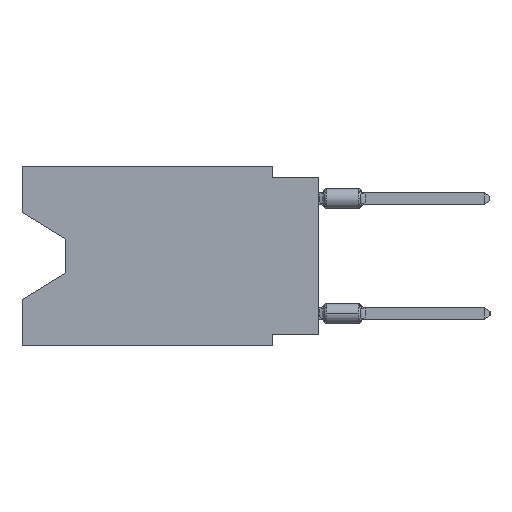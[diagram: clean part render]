
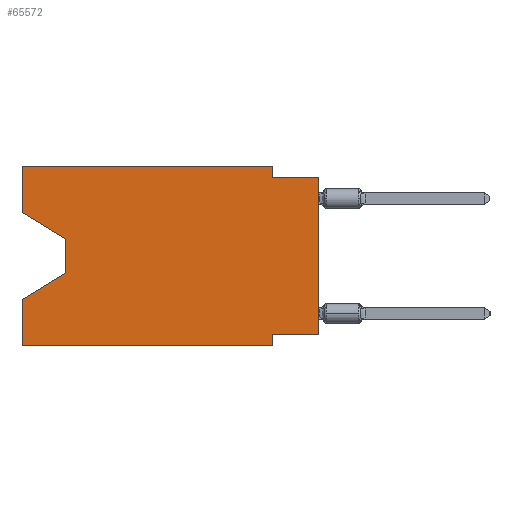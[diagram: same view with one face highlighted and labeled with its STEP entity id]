
A CAD part, left-side view. The second image highlights one B-rep face of the part: STEP entity #65572.
In plain terms, the highlighted planar face has unit normal (-1, 0, 0).
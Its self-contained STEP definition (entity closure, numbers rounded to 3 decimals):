
#178 = VERTEX_POINT ( 'NONE', #41711 ) ;
#434 = EDGE_LOOP ( 'NONE', ( #45684, #6684, #26551, #58628, #59615, #11259, #57603, #14913, #14686, #62036, #37159, #50670 ) ) ;
#535 = VECTOR ( 'NONE', #15756, 1000. ) ;
#4639 = CARTESIAN_POINT ( 'NONE',  ( 0., 2.54, -9.906 ) ) ;
#4961 = VERTEX_POINT ( 'NONE', #57765 ) ;
#5822 = LINE ( 'NONE', #10524, #52215 ) ;
#6130 = VECTOR ( 'NONE', #61492, 1000. ) ;
#6453 = EDGE_CURVE ( 'NONE', #56384, #14442, #25239, .T. ) ;
#6616 = DIRECTION ( 'NONE',  ( 0., 0., 1. ) ) ;
#6684 = ORIENTED_EDGE ( 'NONE', *, *, #17452, .T. ) ;
#6931 = VECTOR ( 'NONE', #47889, 1000. ) ;
#8905 = LINE ( 'NONE', #34385, #12551 ) ;
#10524 = CARTESIAN_POINT ( 'NONE',  ( 0., 16.383, 0. ) ) ;
#11259 = ORIENTED_EDGE ( 'NONE', *, *, #6453, .F. ) ;
#12551 = VECTOR ( 'NONE', #44759, 1000. ) ;
#14379 = VECTOR ( 'NONE', #50388, 1000. ) ;
#14442 = VERTEX_POINT ( 'NONE', #4639 ) ;
#14477 = DIRECTION ( 'NONE',  ( 1., 0., 0. ) ) ;
#14686 = ORIENTED_EDGE ( 'NONE', *, *, #37197, .F. ) ;
#14913 = ORIENTED_EDGE ( 'NONE', *, *, #18314, .T. ) ;
#15156 = EDGE_CURVE ( 'NONE', #62405, #14442, #58585, .T. ) ;
#15756 = DIRECTION ( 'NONE',  ( 0., -0.855, -0.519 ) ) ;
#15877 = DIRECTION ( 'NONE',  ( 0., 0., 1. ) ) ;
#17452 = EDGE_CURVE ( 'NONE', #178, #46009, #27142, .T. ) ;
#17463 = VECTOR ( 'NONE', #6616, 1000. ) ;
#18109 = EDGE_CURVE ( 'NONE', #46009, #28885, #8905, .T. ) ;
#18314 = EDGE_CURVE ( 'NONE', #55580, #65792, #21936, .T. ) ;
#18343 = CARTESIAN_POINT ( 'NONE',  ( 0., 16.383, 0. ) ) ;
#20516 = DIRECTION ( 'NONE',  ( 0., 0., -1. ) ) ;
#21173 = VERTEX_POINT ( 'NONE', #26795 ) ;
#21936 = LINE ( 'NONE', #31014, #6130 ) ;
#22199 = EDGE_CURVE ( 'NONE', #33017, #21173, #59410, .T. ) ;
#23443 = EDGE_CURVE ( 'NONE', #57214, #178, #41226, .T. ) ;
#24512 = VECTOR ( 'NONE', #20516, 1000. ) ;
#25239 = LINE ( 'NONE', #62047, #24512 ) ;
#25458 = CARTESIAN_POINT ( 'NONE',  ( 0., 2.54, 0. ) ) ;
#25638 = CARTESIAN_POINT ( 'NONE',  ( 0., 16.383, -9.906 ) ) ;
#26440 = CARTESIAN_POINT ( 'NONE',  ( 0., 16.383, -7.36 ) ) ;
#26551 = ORIENTED_EDGE ( 'NONE', *, *, #18109, .T. ) ;
#26795 = CARTESIAN_POINT ( 'NONE',  ( 0., 2.54, 0. ) ) ;
#27142 = LINE ( 'NONE', #31824, #30812 ) ;
#28885 = VERTEX_POINT ( 'NONE', #26440 ) ;
#29266 = CARTESIAN_POINT ( 'NONE',  ( 0., 16.383, 0. ) ) ;
#30488 = LINE ( 'NONE', #25458, #59385 ) ;
#30620 = DIRECTION ( 'NONE',  ( 0., -1., 0. ) ) ;
#30709 = CARTESIAN_POINT ( 'NONE',  ( 0., 2.54, -9.271 ) ) ;
#30812 = VECTOR ( 'NONE', #47907, 1000. ) ;
#31014 = CARTESIAN_POINT ( 'NONE',  ( 0., 0., 0. ) ) ;
#31824 = CARTESIAN_POINT ( 'NONE',  ( 0., 13.97, -4.013 ) ) ;
#33017 = VERTEX_POINT ( 'NONE', #18343 ) ;
#33186 = VECTOR ( 'NONE', #30620, 1000. ) ;
#34385 = CARTESIAN_POINT ( 'NONE',  ( 0., 13.97, -5.893 ) ) ;
#36876 = CARTESIAN_POINT ( 'NONE',  ( 0., 0., -0.635 ) ) ;
#37159 = ORIENTED_EDGE ( 'NONE', *, *, #22199, .F. ) ;
#37197 = EDGE_CURVE ( 'NONE', #4961, #65792, #61743, .T. ) ;
#37778 = CARTESIAN_POINT ( 'NONE',  ( 0., 16.383, 0. ) ) ;
#40030 = CARTESIAN_POINT ( 'NONE',  ( 0., 13.97, -5.893 ) ) ;
#41226 = LINE ( 'NONE', #42213, #535 ) ;
#41711 = CARTESIAN_POINT ( 'NONE',  ( 0., 13.97, -4.013 ) ) ;
#42213 = CARTESIAN_POINT ( 'NONE',  ( 0., 16.383, -2.546 ) ) ;
#42941 = EDGE_CURVE ( 'NONE', #62405, #28885, #47854, .T. ) ;
#43161 = CARTESIAN_POINT ( 'NONE',  ( 0., 16.383, -9.906 ) ) ;
#43552 = LINE ( 'NONE', #48283, #52958 ) ;
#44759 = DIRECTION ( 'NONE',  ( 0., 0.855, -0.519 ) ) ;
#45684 = ORIENTED_EDGE ( 'NONE', *, *, #23443, .T. ) ;
#45758 = AXIS2_PLACEMENT_3D ( 'NONE', #61035, #14477, #61369 ) ;
#46009 = VERTEX_POINT ( 'NONE', #40030 ) ;
#47610 = EDGE_CURVE ( 'NONE', #57214, #33017, #5822, .T. ) ;
#47854 = LINE ( 'NONE', #37778, #17463 ) ;
#47889 = DIRECTION ( 'NONE',  ( 0., -1., 0. ) ) ;
#47907 = DIRECTION ( 'NONE',  ( 0., 0., -1. ) ) ;
#48283 = CARTESIAN_POINT ( 'NONE',  ( 0., 0., -9.271 ) ) ;
#50388 = DIRECTION ( 'NONE',  ( 0., -1., 0. ) ) ;
#50670 = ORIENTED_EDGE ( 'NONE', *, *, #47610, .F. ) ;
#50745 = CARTESIAN_POINT ( 'NONE',  ( 0., 0., -0.635 ) ) ;
#51394 = EDGE_CURVE ( 'NONE', #55580, #56384, #43552, .T. ) ;
#51637 = EDGE_CURVE ( 'NONE', #21173, #4961, #30488, .T. ) ;
#52215 = VECTOR ( 'NONE', #15877, 1000. ) ;
#52958 = VECTOR ( 'NONE', #63985, 1000. ) ;
#55580 = VERTEX_POINT ( 'NONE', #57301 ) ;
#55696 = PLANE ( 'NONE',  #45758 ) ;
#56384 = VERTEX_POINT ( 'NONE', #30709 ) ;
#56904 = CARTESIAN_POINT ( 'NONE',  ( 0., 16.383, -2.546 ) ) ;
#57214 = VERTEX_POINT ( 'NONE', #56904 ) ;
#57301 = CARTESIAN_POINT ( 'NONE',  ( 0., 0., -9.271 ) ) ;
#57603 = ORIENTED_EDGE ( 'NONE', *, *, #51394, .F. ) ;
#57765 = CARTESIAN_POINT ( 'NONE',  ( 0., 2.54, -0.635 ) ) ;
#58585 = LINE ( 'NONE', #43161, #6931 ) ;
#58628 = ORIENTED_EDGE ( 'NONE', *, *, #42941, .F. ) ;
#59385 = VECTOR ( 'NONE', #61283, 1000. ) ;
#59410 = LINE ( 'NONE', #29266, #14379 ) ;
#59615 = ORIENTED_EDGE ( 'NONE', *, *, #15156, .T. ) ;
#60705 = FACE_OUTER_BOUND ( 'NONE', #434, .T. ) ;
#61035 = CARTESIAN_POINT ( 'NONE',  ( 0., 16.383, 0. ) ) ;
#61283 = DIRECTION ( 'NONE',  ( 0., 0., -1. ) ) ;
#61369 = DIRECTION ( 'NONE',  ( 0., 0., -1. ) ) ;
#61492 = DIRECTION ( 'NONE',  ( 0., 0., 1. ) ) ;
#61743 = LINE ( 'NONE', #50745, #33186 ) ;
#62036 = ORIENTED_EDGE ( 'NONE', *, *, #51637, .F. ) ;
#62047 = CARTESIAN_POINT ( 'NONE',  ( 0., 2.54, -9.906 ) ) ;
#62405 = VERTEX_POINT ( 'NONE', #25638 ) ;
#63985 = DIRECTION ( 'NONE',  ( 0., 1., 0. ) ) ;
#65572 = ADVANCED_FACE ( 'NONE', ( #60705 ), #55696, .F. ) ;
#65792 = VERTEX_POINT ( 'NONE', #36876 ) ;
